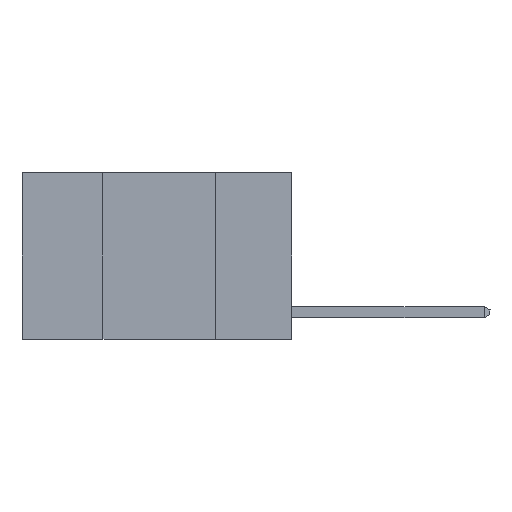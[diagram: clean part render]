
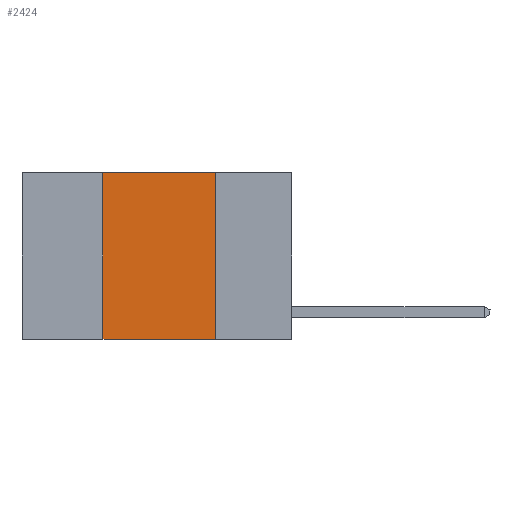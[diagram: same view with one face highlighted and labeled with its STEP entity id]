
A CAD part, left-side view. The second image highlights one B-rep face of the part: STEP entity #2424.
In plain terms, the highlighted planar face has unit normal (-1, 0, 0).
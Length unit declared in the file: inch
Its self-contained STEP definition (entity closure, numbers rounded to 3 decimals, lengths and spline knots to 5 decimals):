
#148 = LINE ( 'NONE', #16375, #18453 ) ;
#2278 = CARTESIAN_POINT ( 'NONE',  ( 0., 0.17, 0. ) ) ;
#2424 = ADVANCED_FACE ( 'NONE', ( #4740 ), #3364, .F. ) ;
#3162 = ORIENTED_EDGE ( 'NONE', *, *, #20562, .F. ) ;
#3364 = PLANE ( 'NONE',  #20010 ) ;
#3569 = EDGE_CURVE ( 'NONE', #13774, #11297, #15920, .T. ) ;
#3904 = ORIENTED_EDGE ( 'NONE', *, *, #3569, .F. ) ;
#4682 = DIRECTION ( 'NONE',  ( 0., 0., -1. ) ) ;
#4740 = FACE_OUTER_BOUND ( 'NONE', #24293, .T. ) ;
#5687 = LINE ( 'NONE', #2278, #17623 ) ;
#8145 = DIRECTION ( 'NONE',  ( 0., 0., -1. ) ) ;
#8861 = VERTEX_POINT ( 'NONE', #11064 ) ;
#9192 = LINE ( 'NONE', #21020, #21152 ) ;
#10245 = CARTESIAN_POINT ( 'NONE',  ( 0., 0.6, 0. ) ) ;
#11064 = CARTESIAN_POINT ( 'NONE',  ( 0., 0.42, -0.37 ) ) ;
#11297 = VERTEX_POINT ( 'NONE', #25580 ) ;
#11979 = CARTESIAN_POINT ( 'NONE',  ( 0., 0.17, -0.37 ) ) ;
#12725 = EDGE_CURVE ( 'NONE', #8861, #30800, #9192, .T. ) ;
#13774 = VERTEX_POINT ( 'NONE', #22214 ) ;
#15064 = DIRECTION ( 'NONE',  ( 0., -1., 0. ) ) ;
#15235 = CARTESIAN_POINT ( 'NONE',  ( 0., 0.6, 0. ) ) ;
#15920 = LINE ( 'NONE', #10245, #22250 ) ;
#16375 = CARTESIAN_POINT ( 'NONE',  ( 0., 0.42, 0. ) ) ;
#17623 = VECTOR ( 'NONE', #4682, 39.37008 ) ;
#18111 = ORIENTED_EDGE ( 'NONE', *, *, #12725, .T. ) ;
#18453 = VECTOR ( 'NONE', #18792, 39.37008 ) ;
#18555 = EDGE_CURVE ( 'NONE', #8861, #13774, #148, .T. ) ;
#18792 = DIRECTION ( 'NONE',  ( 0., 0., 1. ) ) ;
#20010 = AXIS2_PLACEMENT_3D ( 'NONE', #15235, #22428, #8145 ) ;
#20562 = EDGE_CURVE ( 'NONE', #11297, #30800, #5687, .T. ) ;
#21020 = CARTESIAN_POINT ( 'NONE',  ( 0., 0.6, -0.37 ) ) ;
#21152 = VECTOR ( 'NONE', #25805, 39.37008 ) ;
#22214 = CARTESIAN_POINT ( 'NONE',  ( 0., 0.42, 0. ) ) ;
#22250 = VECTOR ( 'NONE', #15064, 39.37008 ) ;
#22428 = DIRECTION ( 'NONE',  ( 1., 0., 0. ) ) ;
#24293 = EDGE_LOOP ( 'NONE', ( #3162, #3904, #29966, #18111 ) ) ;
#25580 = CARTESIAN_POINT ( 'NONE',  ( 0., 0.17, 0. ) ) ;
#25805 = DIRECTION ( 'NONE',  ( 0., -1., 0. ) ) ;
#29966 = ORIENTED_EDGE ( 'NONE', *, *, #18555, .F. ) ;
#30800 = VERTEX_POINT ( 'NONE', #11979 ) ;
